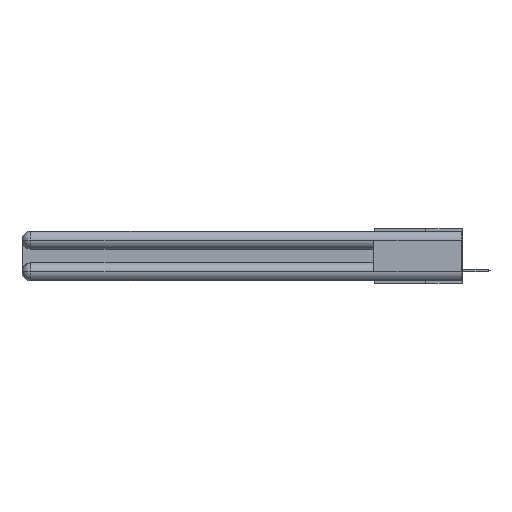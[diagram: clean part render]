
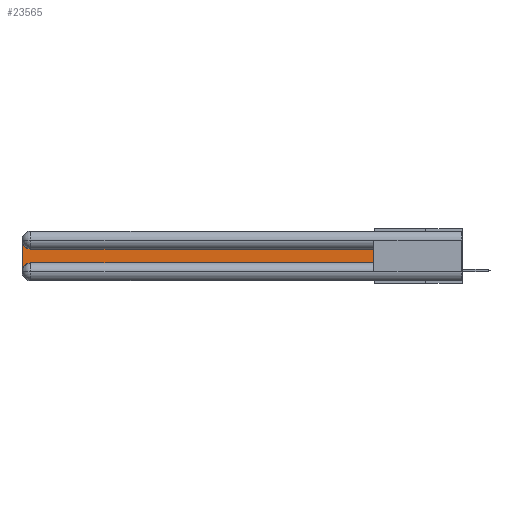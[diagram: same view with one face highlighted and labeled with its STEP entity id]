
A CAD part, left-side view. The second image highlights one B-rep face of the part: STEP entity #23565.
In plain terms, the highlighted planar face has unit normal (-1, 0, 0).
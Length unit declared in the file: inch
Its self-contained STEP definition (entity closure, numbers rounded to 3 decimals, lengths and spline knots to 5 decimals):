
#7 = VECTOR ( 'NONE', #19305, 39.37008 ) ;
#799 = DIRECTION ( 'NONE',  ( 0., 0., -1. ) ) ;
#1074 = CARTESIAN_POINT ( 'NONE',  ( 0.075, 0.6, -0.2175 ) ) ;
#1592 = EDGE_CURVE ( 'NONE', #24515, #12571, #15310, .T. ) ;
#2816 = EDGE_CURVE ( 'NONE', #24072, #4994, #10331, .T. ) ;
#4335 = AXIS2_PLACEMENT_3D ( 'NONE', #8669, #26719, #799 ) ;
#4994 = VERTEX_POINT ( 'NONE', #24578 ) ;
#5110 = CARTESIAN_POINT ( 'NONE',  ( 0.075, 3., -0.2175 ) ) ;
#6578 = DIRECTION ( 'NONE',  ( 0., 0., -1. ) ) ;
#8669 = CARTESIAN_POINT ( 'NONE',  ( 0.075, 2.94, -0.2775 ) ) ;
#8685 = EDGE_CURVE ( 'NONE', #25216, #24515, #22437, .T. ) ;
#8731 = CARTESIAN_POINT ( 'NONE',  ( 0.075, 0.6, -0.1225 ) ) ;
#8892 = ORIENTED_EDGE ( 'NONE', *, *, #28922, .T. ) ;
#8990 = VECTOR ( 'NONE', #21008, 39.37008 ) ;
#10208 = CARTESIAN_POINT ( 'NONE',  ( 0.075, 2.94, -0.0625 ) ) ;
#10319 = DIRECTION ( 'NONE',  ( 0., 0., -1. ) ) ;
#10331 = CIRCLE ( 'NONE', #13690, 0.06 ) ;
#10420 = CARTESIAN_POINT ( 'NONE',  ( 0.075, 2.94, -0.2175 ) ) ;
#10611 = CARTESIAN_POINT ( 'NONE',  ( 0.075, 2.94, -0.1225 ) ) ;
#12517 = FACE_OUTER_BOUND ( 'NONE', #24892, .T. ) ;
#12571 = VERTEX_POINT ( 'NONE', #14382 ) ;
#12709 = VERTEX_POINT ( 'NONE', #17323 ) ;
#13690 = AXIS2_PLACEMENT_3D ( 'NONE', #10208, #25563, #10319 ) ;
#14131 = DIRECTION ( 'NONE',  ( 1., 0., 0. ) ) ;
#14382 = CARTESIAN_POINT ( 'NONE',  ( 0.075, 0.6, -0.2175 ) ) ;
#14672 = ORIENTED_EDGE ( 'NONE', *, *, #1592, .T. ) ;
#15310 = LINE ( 'NONE', #16932, #7 ) ;
#16932 = CARTESIAN_POINT ( 'NONE',  ( 0.075, 0.6, -0.2175 ) ) ;
#17174 = ORIENTED_EDGE ( 'NONE', *, *, #31464, .T. ) ;
#17323 = CARTESIAN_POINT ( 'NONE',  ( 0.075, 0.6, -0.1225 ) ) ;
#19305 = DIRECTION ( 'NONE',  ( 0., -1., 0. ) ) ;
#19345 = PLANE ( 'NONE',  #31510 ) ;
#21008 = DIRECTION ( 'NONE',  ( 0., 0., 1. ) ) ;
#22027 = CARTESIAN_POINT ( 'NONE',  ( 0.075, 3., -0.1225 ) ) ;
#22437 = CIRCLE ( 'NONE', #4335, 0.06 ) ;
#22674 = VECTOR ( 'NONE', #29332, 39.37008 ) ;
#23199 = LINE ( 'NONE', #5110, #30447 ) ;
#23565 = ADVANCED_FACE ( 'NONE', ( #12517 ), #19345, .F. ) ;
#23623 = CARTESIAN_POINT ( 'NONE',  ( 0.075, 3., -0.2775 ) ) ;
#23835 = ORIENTED_EDGE ( 'NONE', *, *, #2816, .T. ) ;
#24072 = VERTEX_POINT ( 'NONE', #10611 ) ;
#24515 = VERTEX_POINT ( 'NONE', #10420 ) ;
#24578 = CARTESIAN_POINT ( 'NONE',  ( 0.075, 3., -0.0625 ) ) ;
#24892 = EDGE_LOOP ( 'NONE', ( #17174, #23835, #8892, #31593, #14672, #30745 ) ) ;
#25216 = VERTEX_POINT ( 'NONE', #23623 ) ;
#25563 = DIRECTION ( 'NONE',  ( 1., 0., 0. ) ) ;
#26331 = LINE ( 'NONE', #1074, #8990 ) ;
#26686 = LINE ( 'NONE', #8731, #22674 ) ;
#26719 = DIRECTION ( 'NONE',  ( 1., 0., 0. ) ) ;
#28922 = EDGE_CURVE ( 'NONE', #4994, #25216, #23199, .T. ) ;
#29332 = DIRECTION ( 'NONE',  ( 0., 1., 0. ) ) ;
#30447 = VECTOR ( 'NONE', #30919, 39.37008 ) ;
#30745 = ORIENTED_EDGE ( 'NONE', *, *, #32987, .T. ) ;
#30919 = DIRECTION ( 'NONE',  ( 0., 0., -1. ) ) ;
#31464 = EDGE_CURVE ( 'NONE', #12709, #24072, #26686, .T. ) ;
#31510 = AXIS2_PLACEMENT_3D ( 'NONE', #22027, #14131, #6578 ) ;
#31593 = ORIENTED_EDGE ( 'NONE', *, *, #8685, .T. ) ;
#32987 = EDGE_CURVE ( 'NONE', #12571, #12709, #26331, .T. ) ;
